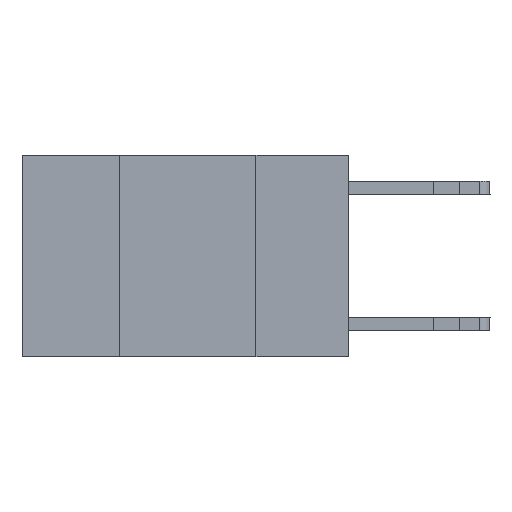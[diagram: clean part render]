
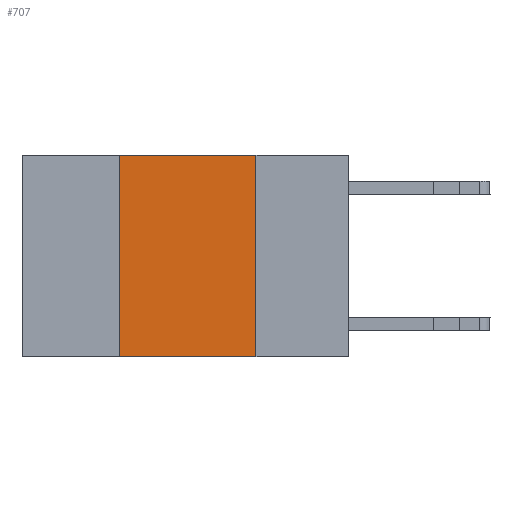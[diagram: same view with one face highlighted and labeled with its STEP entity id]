
A CAD part, left-side view. The second image highlights one B-rep face of the part: STEP entity #707.
In plain terms, the highlighted planar face has unit normal (-1, 0, 0).
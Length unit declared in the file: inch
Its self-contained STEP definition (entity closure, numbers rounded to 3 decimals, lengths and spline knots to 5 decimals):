
#124 = LINE ( 'NONE', #3612, #10716 ) ;
#707 = ADVANCED_FACE ( 'NONE', ( #3564 ), #4858, .F. ) ;
#790 = CARTESIAN_POINT ( 'NONE',  ( 0., 0.17, -0.37 ) ) ;
#1827 = CARTESIAN_POINT ( 'NONE',  ( 0., 0.6, -0.37 ) ) ;
#2263 = CARTESIAN_POINT ( 'NONE',  ( 0., 0.6, 0. ) ) ;
#2411 = ORIENTED_EDGE ( 'NONE', *, *, #9984, .F. ) ;
#2951 = LINE ( 'NONE', #1827, #10185 ) ;
#3564 = FACE_OUTER_BOUND ( 'NONE', #5382, .T. ) ;
#3612 = CARTESIAN_POINT ( 'NONE',  ( 0., 0.6, 0. ) ) ;
#3885 = CARTESIAN_POINT ( 'NONE',  ( 0., 0.17, 0. ) ) ;
#4178 = DIRECTION ( 'NONE',  ( 0., -1., 0. ) ) ;
#4529 = LINE ( 'NONE', #14408, #8212 ) ;
#4808 = DIRECTION ( 'NONE',  ( 0., 0., -1. ) ) ;
#4858 = PLANE ( 'NONE',  #9145 ) ;
#5005 = DIRECTION ( 'NONE',  ( 1., 0., 0. ) ) ;
#5107 = LINE ( 'NONE', #3885, #13883 ) ;
#5382 = EDGE_LOOP ( 'NONE', ( #8855, #2411, #14983, #9386 ) ) ;
#6120 = DIRECTION ( 'NONE',  ( 0., -1., 0. ) ) ;
#6878 = EDGE_CURVE ( 'NONE', #13044, #11088, #2951, .T. ) ;
#7021 = DIRECTION ( 'NONE',  ( 0., 0., 1. ) ) ;
#7024 = VERTEX_POINT ( 'NONE', #15613 ) ;
#8165 = CARTESIAN_POINT ( 'NONE',  ( 0., 0.17, 0. ) ) ;
#8212 = VECTOR ( 'NONE', #7021, 39.37008 ) ;
#8855 = ORIENTED_EDGE ( 'NONE', *, *, #9180, .F. ) ;
#9048 = CARTESIAN_POINT ( 'NONE',  ( 0., 0.42, -0.37 ) ) ;
#9145 = AXIS2_PLACEMENT_3D ( 'NONE', #2263, #5005, #10947 ) ;
#9180 = EDGE_CURVE ( 'NONE', #13310, #11088, #5107, .T. ) ;
#9386 = ORIENTED_EDGE ( 'NONE', *, *, #6878, .T. ) ;
#9984 = EDGE_CURVE ( 'NONE', #7024, #13310, #124, .T. ) ;
#10185 = VECTOR ( 'NONE', #4178, 39.37008 ) ;
#10716 = VECTOR ( 'NONE', #6120, 39.37008 ) ;
#10947 = DIRECTION ( 'NONE',  ( 0., 0., -1. ) ) ;
#11088 = VERTEX_POINT ( 'NONE', #790 ) ;
#13044 = VERTEX_POINT ( 'NONE', #9048 ) ;
#13310 = VERTEX_POINT ( 'NONE', #8165 ) ;
#13883 = VECTOR ( 'NONE', #4808, 39.37008 ) ;
#14143 = EDGE_CURVE ( 'NONE', #13044, #7024, #4529, .T. ) ;
#14408 = CARTESIAN_POINT ( 'NONE',  ( 0., 0.42, 0. ) ) ;
#14983 = ORIENTED_EDGE ( 'NONE', *, *, #14143, .F. ) ;
#15613 = CARTESIAN_POINT ( 'NONE',  ( 0., 0.42, 0. ) ) ;
